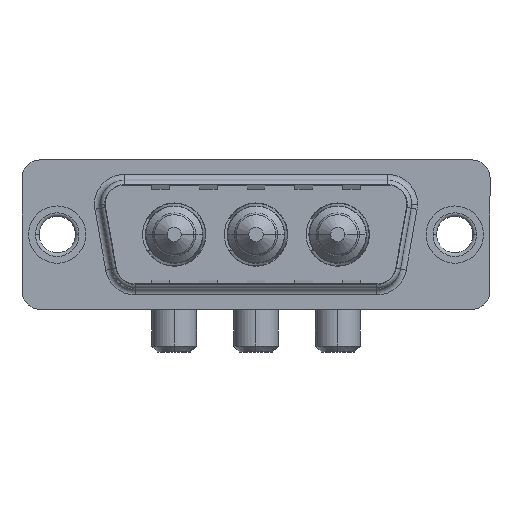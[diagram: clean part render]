
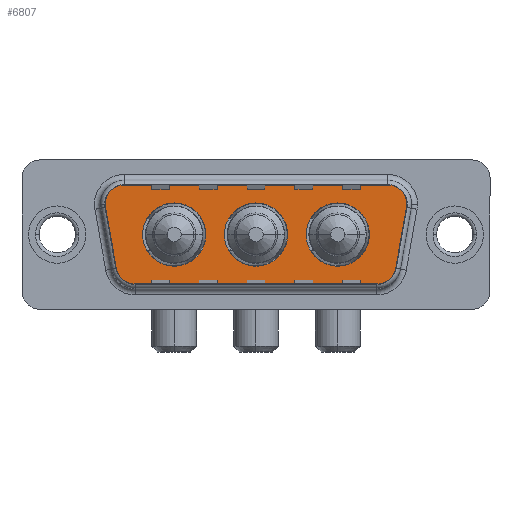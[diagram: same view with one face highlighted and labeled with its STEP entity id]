
A CAD part, top view. The second image highlights one B-rep face of the part: STEP entity #6807.
In plain terms, the highlighted planar face has unit normal (0, 0, 1).
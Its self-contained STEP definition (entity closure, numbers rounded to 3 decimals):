
#179 = ORIENTED_EDGE ( 'NONE', *, *, #8865, .T. ) ;
#185 = DIRECTION ( 'NONE',  ( -1., 0., 0. ) ) ;
#520 = EDGE_CURVE ( 'NONE', #6332, #8855, #4629, .T. ) ;
#882 = DIRECTION ( 'NONE',  ( 0., 0., 1. ) ) ;
#1051 = CARTESIAN_POINT ( 'NONE',  ( 29.859, 2.553, 0. ) ) ;
#1058 = DIRECTION ( 'NONE',  ( 0., 0., 1. ) ) ;
#1070 = CARTESIAN_POINT ( 'NONE',  ( 4.464, -3.247, 0. ) ) ;
#1175 = DIRECTION ( 'NONE',  ( 1., 0., 0. ) ) ;
#1533 = CIRCLE ( 'NONE', #4049, 2.65 ) ;
#1549 = CARTESIAN_POINT ( 'NONE',  ( 29.859, 2.553, 0. ) ) ;
#1556 = LINE ( 'NONE', #2295, #4862 ) ;
#1592 = DIRECTION ( 'NONE',  ( 1., 0., 0. ) ) ;
#1799 = AXIS2_PLACEMENT_3D ( 'NONE', #8750, #1058, #9642 ) ;
#1975 = VERTEX_POINT ( 'NONE', #7512 ) ;
#2107 = EDGE_LOOP ( 'NONE', ( #4645, #4354 ) ) ;
#2128 = DIRECTION ( 'NONE',  ( 0., 0., 1. ) ) ;
#2144 = CARTESIAN_POINT ( 'NONE',  ( 6.434, -4.9, 0. ) ) ;
#2278 = DIRECTION ( 'NONE',  ( 0., 0., 1. ) ) ;
#2295 = CARTESIAN_POINT ( 'NONE',  ( 3.441, 2.553, 0. ) ) ;
#2320 = PLANE ( 'NONE',  #10064 ) ;
#2523 = AXIS2_PLACEMENT_3D ( 'NONE', #4014, #5075, #3227 ) ;
#2561 = DIRECTION ( 'NONE',  ( 1., 0., 0. ) ) ;
#2571 = EDGE_CURVE ( 'NONE', #8984, #8884, #1533, .T. ) ;
#2624 = DIRECTION ( 'NONE',  ( 1., 0., 0. ) ) ;
#3046 = EDGE_LOOP ( 'NONE', ( #3744, #6493, #3312, #6589, #9756, #9444, #7386, #179, #5580 ) ) ;
#3064 = DIRECTION ( 'NONE',  ( 0., 0., 1. ) ) ;
#3127 = DIRECTION ( 'NONE',  ( 0., 0., 1. ) ) ;
#3227 = DIRECTION ( 'NONE',  ( -1., 0., 0. ) ) ;
#3248 = DIRECTION ( 'NONE',  ( 0.174, -0.985, 0. ) ) ;
#3312 = ORIENTED_EDGE ( 'NONE', *, *, #3971, .T. ) ;
#3418 = AXIS2_PLACEMENT_3D ( 'NONE', #7594, #3127, #10799 ) ;
#3616 = DIRECTION ( 'NONE',  ( 1., 0., 0. ) ) ;
#3626 = LINE ( 'NONE', #5306, #4981 ) ;
#3742 = AXIS2_PLACEMENT_3D ( 'NONE', #6372, #3064, #7321 ) ;
#3744 = ORIENTED_EDGE ( 'NONE', *, *, #6305, .T. ) ;
#3750 = EDGE_LOOP ( 'NONE', ( #4702, #8488 ) ) ;
#3824 = CIRCLE ( 'NONE', #3991, 2.65 ) ;
#3971 = EDGE_CURVE ( 'NONE', #6058, #1975, #8419, .T. ) ;
#3991 = AXIS2_PLACEMENT_3D ( 'NONE', #5270, #882, #2561 ) ;
#4006 = FACE_BOUND ( 'NONE', #9952, .T. ) ;
#4014 = CARTESIAN_POINT ( 'NONE',  ( 27.889, 2.9, 0. ) ) ;
#4015 = EDGE_CURVE ( 'NONE', #8227, #7709, #4312, .T. ) ;
#4049 = AXIS2_PLACEMENT_3D ( 'NONE', #4646, #8062, #8000 ) ;
#4060 = CARTESIAN_POINT ( 'NONE',  ( 19.3, 0., 0. ) ) ;
#4071 = AXIS2_PLACEMENT_3D ( 'NONE', #6384, #9739, #9858 ) ;
#4152 = EDGE_CURVE ( 'NONE', #4563, #8058, #4482, .T. ) ;
#4168 = FACE_BOUND ( 'NONE', #3750, .T. ) ;
#4312 = CIRCLE ( 'NONE', #8789, 2.65 ) ;
#4342 = EDGE_CURVE ( 'NONE', #7709, #8227, #7188, .T. ) ;
#4354 = ORIENTED_EDGE ( 'NONE', *, *, #520, .F. ) ;
#4355 = VECTOR ( 'NONE', #3616, 1000. ) ;
#4446 = CARTESIAN_POINT ( 'NONE',  ( 27.889, 4.9, 0. ) ) ;
#4449 = CARTESIAN_POINT ( 'NONE',  ( 6.434, -4.9, 0. ) ) ;
#4482 = CIRCLE ( 'NONE', #5021, 2. ) ;
#4544 = EDGE_CURVE ( 'NONE', #10590, #6058, #10967, .T. ) ;
#4563 = VERTEX_POINT ( 'NONE', #5984 ) ;
#4629 = CIRCLE ( 'NONE', #10167, 2.65 ) ;
#4633 = CIRCLE ( 'NONE', #3742, 2. ) ;
#4645 = ORIENTED_EDGE ( 'NONE', *, *, #9680, .F. ) ;
#4646 = CARTESIAN_POINT ( 'NONE',  ( 16.65, 0., 0. ) ) ;
#4702 = ORIENTED_EDGE ( 'NONE', *, *, #2571, .F. ) ;
#4714 = CARTESIAN_POINT ( 'NONE',  ( 23.5, 0., 0. ) ) ;
#4862 = VECTOR ( 'NONE', #3248, 1000. ) ;
#4897 = CARTESIAN_POINT ( 'NONE',  ( 26.866, -2.9, 0. ) ) ;
#4981 = VECTOR ( 'NONE', #185, 1000. ) ;
#4996 = EDGE_CURVE ( 'NONE', #1975, #9124, #7369, .T. ) ;
#5021 = AXIS2_PLACEMENT_3D ( 'NONE', #5894, #8579, #2624 ) ;
#5075 = DIRECTION ( 'NONE',  ( 0., 0., 1. ) ) ;
#5270 = CARTESIAN_POINT ( 'NONE',  ( 16.65, 0., 0. ) ) ;
#5306 = CARTESIAN_POINT ( 'NONE',  ( 5.411, 4.9, 0. ) ) ;
#5373 = VERTEX_POINT ( 'NONE', #2144 ) ;
#5580 = ORIENTED_EDGE ( 'NONE', *, *, #10369, .T. ) ;
#5611 = VERTEX_POINT ( 'NONE', #1070 ) ;
#5830 = CARTESIAN_POINT ( 'NONE',  ( 12.45, 0., 0. ) ) ;
#5894 = CARTESIAN_POINT ( 'NONE',  ( 5.411, 2.9, 0. ) ) ;
#5984 = CARTESIAN_POINT ( 'NONE',  ( 5.411, 4.9, 0. ) ) ;
#6058 = VERTEX_POINT ( 'NONE', #1051 ) ;
#6305 = EDGE_CURVE ( 'NONE', #6445, #10590, #8195, .T. ) ;
#6332 = VERTEX_POINT ( 'NONE', #9799 ) ;
#6372 = CARTESIAN_POINT ( 'NONE',  ( 6.434, -2.9, 0. ) ) ;
#6384 = CARTESIAN_POINT ( 'NONE',  ( 26.866, -2.9, 0. ) ) ;
#6403 = CARTESIAN_POINT ( 'NONE',  ( 23.5, 0., 0. ) ) ;
#6445 = VERTEX_POINT ( 'NONE', #8437 ) ;
#6493 = ORIENTED_EDGE ( 'NONE', *, *, #4544, .T. ) ;
#6582 = FACE_BOUND ( 'NONE', #2107, .T. ) ;
#6589 = ORIENTED_EDGE ( 'NONE', *, *, #4996, .T. ) ;
#6807 = ADVANCED_FACE ( 'NONE', ( #4168, #6582, #4006, #7420 ), #2320, .T. ) ;
#7188 = CIRCLE ( 'NONE', #1799, 2.65 ) ;
#7321 = DIRECTION ( 'NONE',  ( -1., 0., 0. ) ) ;
#7369 = CIRCLE ( 'NONE', #2523, 2. ) ;
#7386 = ORIENTED_EDGE ( 'NONE', *, *, #7687, .T. ) ;
#7420 = FACE_OUTER_BOUND ( 'NONE', #3046, .T. ) ;
#7512 = CARTESIAN_POINT ( 'NONE',  ( 29.889, 2.9, 0. ) ) ;
#7559 = CIRCLE ( 'NONE', #8640, 2.65 ) ;
#7594 = CARTESIAN_POINT ( 'NONE',  ( 27.889, 2.9, 0. ) ) ;
#7687 = EDGE_CURVE ( 'NONE', #8058, #5611, #1556, .T. ) ;
#7709 = VERTEX_POINT ( 'NONE', #5830 ) ;
#8000 = DIRECTION ( 'NONE',  ( 1., 0., 0. ) ) ;
#8039 = CARTESIAN_POINT ( 'NONE',  ( 28.836, -3.247, 0. ) ) ;
#8058 = VERTEX_POINT ( 'NONE', #10679 ) ;
#8062 = DIRECTION ( 'NONE',  ( 0., 0., 1. ) ) ;
#8136 = DIRECTION ( 'NONE',  ( 1., 0., 0. ) ) ;
#8195 = CIRCLE ( 'NONE', #4071, 2. ) ;
#8227 = VERTEX_POINT ( 'NONE', #9546 ) ;
#8419 = CIRCLE ( 'NONE', #3418, 2. ) ;
#8437 = CARTESIAN_POINT ( 'NONE',  ( 26.866, -4.9, 0. ) ) ;
#8483 = CARTESIAN_POINT ( 'NONE',  ( 14., 0., 0. ) ) ;
#8488 = ORIENTED_EDGE ( 'NONE', *, *, #9931, .F. ) ;
#8579 = DIRECTION ( 'NONE',  ( 0., 0., 1. ) ) ;
#8640 = AXIS2_PLACEMENT_3D ( 'NONE', #4714, #9926, #1175 ) ;
#8653 = EDGE_CURVE ( 'NONE', #9124, #4563, #3626, .T. ) ;
#8750 = CARTESIAN_POINT ( 'NONE',  ( 9.8, 0., 0. ) ) ;
#8789 = AXIS2_PLACEMENT_3D ( 'NONE', #9128, #2278, #1592 ) ;
#8840 = ORIENTED_EDGE ( 'NONE', *, *, #4342, .F. ) ;
#8855 = VERTEX_POINT ( 'NONE', #10625 ) ;
#8865 = EDGE_CURVE ( 'NONE', #5611, #5373, #4633, .T. ) ;
#8884 = VERTEX_POINT ( 'NONE', #8483 ) ;
#8984 = VERTEX_POINT ( 'NONE', #4060 ) ;
#9124 = VERTEX_POINT ( 'NONE', #4446 ) ;
#9128 = CARTESIAN_POINT ( 'NONE',  ( 9.8, 0., 0. ) ) ;
#9444 = ORIENTED_EDGE ( 'NONE', *, *, #4152, .T. ) ;
#9546 = CARTESIAN_POINT ( 'NONE',  ( 7.15, 0., 0. ) ) ;
#9642 = DIRECTION ( 'NONE',  ( 1., 0., 0. ) ) ;
#9680 = EDGE_CURVE ( 'NONE', #8855, #6332, #7559, .T. ) ;
#9739 = DIRECTION ( 'NONE',  ( 0., 0., 1. ) ) ;
#9756 = ORIENTED_EDGE ( 'NONE', *, *, #8653, .T. ) ;
#9799 = CARTESIAN_POINT ( 'NONE',  ( 20.85, 0., 0. ) ) ;
#9858 = DIRECTION ( 'NONE',  ( 1., 0., 0. ) ) ;
#9926 = DIRECTION ( 'NONE',  ( 0., 0., 1. ) ) ;
#9931 = EDGE_CURVE ( 'NONE', #8884, #8984, #3824, .T. ) ;
#9952 = EDGE_LOOP ( 'NONE', ( #8840, #10427 ) ) ;
#10064 = AXIS2_PLACEMENT_3D ( 'NONE', #4897, #10163, #10943 ) ;
#10163 = DIRECTION ( 'NONE',  ( 0., 0., 1. ) ) ;
#10167 = AXIS2_PLACEMENT_3D ( 'NONE', #6403, #2128, #8136 ) ;
#10215 = VECTOR ( 'NONE', #11078, 1000. ) ;
#10369 = EDGE_CURVE ( 'NONE', #5373, #6445, #10440, .T. ) ;
#10427 = ORIENTED_EDGE ( 'NONE', *, *, #4015, .F. ) ;
#10440 = LINE ( 'NONE', #4449, #4355 ) ;
#10590 = VERTEX_POINT ( 'NONE', #8039 ) ;
#10625 = CARTESIAN_POINT ( 'NONE',  ( 26.15, 0., 0. ) ) ;
#10679 = CARTESIAN_POINT ( 'NONE',  ( 3.441, 2.553, 0. ) ) ;
#10799 = DIRECTION ( 'NONE',  ( -1., 0., 0. ) ) ;
#10943 = DIRECTION ( 'NONE',  ( 1., 0., 0. ) ) ;
#10967 = LINE ( 'NONE', #1549, #10215 ) ;
#11078 = DIRECTION ( 'NONE',  ( 0.174, 0.985, 0. ) ) ;
